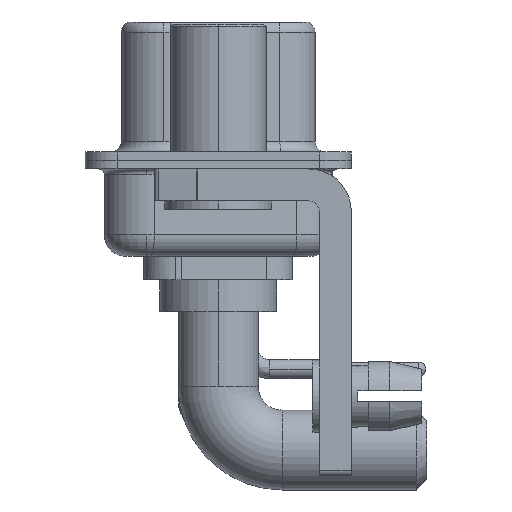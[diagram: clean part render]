
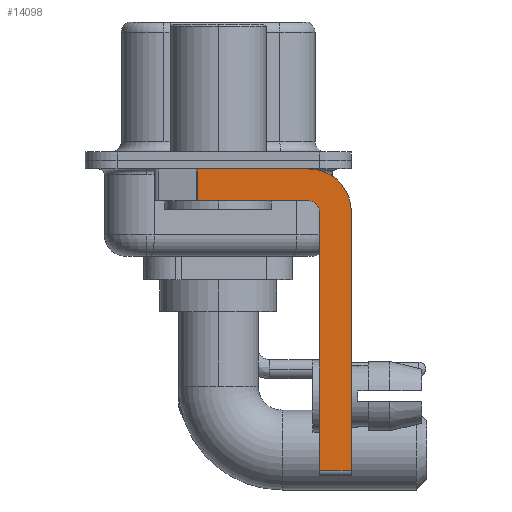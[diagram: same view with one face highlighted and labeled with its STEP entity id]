
A CAD part, left-side view. The second image highlights one B-rep face of the part: STEP entity #14098.
In plain terms, the highlighted planar face has unit normal (-1, 0, 0).
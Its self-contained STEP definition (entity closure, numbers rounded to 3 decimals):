
#633 = VERTEX_POINT ( 'NONE', #11677 ) ;
#775 = EDGE_CURVE ( 'NONE', #2592, #633, #16320, .T. ) ;
#2592 = VERTEX_POINT ( 'NONE', #19763 ) ;
#3270 = CARTESIAN_POINT ( 'NONE',  ( -2.9, -4.75, -2.4 ) ) ;
#3428 = VERTEX_POINT ( 'NONE', #3270 ) ;
#3768 = CARTESIAN_POINT ( 'NONE',  ( -2.9, -4.25, -2.4 ) ) ;
#4276 = EDGE_LOOP ( 'NONE', ( #9326, #21730, #4498, #8214, #5578, #11010, #11119, #6740 ) ) ;
#4498 = ORIENTED_EDGE ( 'NONE', *, *, #6922, .F. ) ;
#4582 = CARTESIAN_POINT ( 'NONE',  ( -2.9, -4.25, -0.4 ) ) ;
#4956 = AXIS2_PLACEMENT_3D ( 'NONE', #20406, #5187, #14983 ) ;
#5001 = CARTESIAN_POINT ( 'NONE',  ( -2.9, 0.978, -1.9 ) ) ;
#5187 = DIRECTION ( 'NONE',  ( -1., 0., 0. ) ) ;
#5353 = LINE ( 'NONE', #20832, #12167 ) ;
#5423 = CARTESIAN_POINT ( 'NONE',  ( -2.9, -4.25, -1.9 ) ) ;
#5578 = ORIENTED_EDGE ( 'NONE', *, *, #13002, .F. ) ;
#5621 = LINE ( 'NONE', #15037, #17516 ) ;
#5906 = PLANE ( 'NONE',  #6589 ) ;
#6129 = CARTESIAN_POINT ( 'NONE',  ( -2.9, -4.25, -2.4 ) ) ;
#6556 = VECTOR ( 'NONE', #11486, 1000. ) ;
#6589 = AXIS2_PLACEMENT_3D ( 'NONE', #3768, #19497, #24944 ) ;
#6740 = ORIENTED_EDGE ( 'NONE', *, *, #20470, .F. ) ;
#6922 = EDGE_CURVE ( 'NONE', #8669, #633, #5353, .T. ) ;
#7540 = LINE ( 'NONE', #13399, #6556 ) ;
#7844 = VECTOR ( 'NONE', #14550, 1000. ) ;
#8214 = ORIENTED_EDGE ( 'NONE', *, *, #13519, .F. ) ;
#8218 = EDGE_CURVE ( 'NONE', #18085, #17598, #7540, .T. ) ;
#8669 = VERTEX_POINT ( 'NONE', #5423 ) ;
#9326 = ORIENTED_EDGE ( 'NONE', *, *, #13284, .F. ) ;
#9470 = FACE_OUTER_BOUND ( 'NONE', #4276, .T. ) ;
#10222 = LINE ( 'NONE', #21998, #17088 ) ;
#10556 = VERTEX_POINT ( 'NONE', #4582 ) ;
#11010 = ORIENTED_EDGE ( 'NONE', *, *, #8218, .T. ) ;
#11119 = ORIENTED_EDGE ( 'NONE', *, *, #16963, .F. ) ;
#11486 = DIRECTION ( 'NONE',  ( 0., -1., 0. ) ) ;
#11677 = CARTESIAN_POINT ( 'NONE',  ( -2.9, 0.978, -1.9 ) ) ;
#12007 = CIRCLE ( 'NONE', #22108, 2. ) ;
#12167 = VECTOR ( 'NONE', #18302, 1000. ) ;
#13002 = EDGE_CURVE ( 'NONE', #18085, #3428, #10222, .T. ) ;
#13284 = EDGE_CURVE ( 'NONE', #2592, #10556, #5621, .T. ) ;
#13399 = CARTESIAN_POINT ( 'NONE',  ( -2.9, -4.25, -14.55 ) ) ;
#13519 = EDGE_CURVE ( 'NONE', #3428, #8669, #15122, .T. ) ;
#13647 = DIRECTION ( 'NONE',  ( 0., 0., -1. ) ) ;
#13901 = DIRECTION ( 'NONE',  ( 1., 0., 0. ) ) ;
#14098 = ADVANCED_FACE ( 'NONE', ( #9470 ), #5906, .F. ) ;
#14173 = DIRECTION ( 'NONE',  ( 0., 0., 1. ) ) ;
#14500 = LINE ( 'NONE', #22211, #17195 ) ;
#14550 = DIRECTION ( 'NONE',  ( 0., 0., -1. ) ) ;
#14983 = DIRECTION ( 'NONE',  ( 0., 0., 1. ) ) ;
#15037 = CARTESIAN_POINT ( 'NONE',  ( -2.9, 3., -0.4 ) ) ;
#15122 = CIRCLE ( 'NONE', #4956, 0.5 ) ;
#16320 = LINE ( 'NONE', #5001, #7844 ) ;
#16439 = VERTEX_POINT ( 'NONE', #16442 ) ;
#16442 = CARTESIAN_POINT ( 'NONE',  ( -2.9, -6.25, -2.4 ) ) ;
#16963 = EDGE_CURVE ( 'NONE', #16439, #17598, #14500, .T. ) ;
#17088 = VECTOR ( 'NONE', #14173, 1000. ) ;
#17135 = DIRECTION ( 'NONE',  ( 0., 0., -1. ) ) ;
#17195 = VECTOR ( 'NONE', #17135, 1000. ) ;
#17516 = VECTOR ( 'NONE', #23265, 1000. ) ;
#17598 = VERTEX_POINT ( 'NONE', #23324 ) ;
#18085 = VERTEX_POINT ( 'NONE', #23426 ) ;
#18302 = DIRECTION ( 'NONE',  ( 0., 1., 0. ) ) ;
#19497 = DIRECTION ( 'NONE',  ( 1., 0., 0. ) ) ;
#19763 = CARTESIAN_POINT ( 'NONE',  ( -2.9, 0.978, -0.4 ) ) ;
#20406 = CARTESIAN_POINT ( 'NONE',  ( -2.9, -4.25, -2.4 ) ) ;
#20470 = EDGE_CURVE ( 'NONE', #10556, #16439, #12007, .T. ) ;
#20832 = CARTESIAN_POINT ( 'NONE',  ( -2.9, -4.25, -1.9 ) ) ;
#21730 = ORIENTED_EDGE ( 'NONE', *, *, #775, .T. ) ;
#21998 = CARTESIAN_POINT ( 'NONE',  ( -2.9, -4.75, -14.8 ) ) ;
#22108 = AXIS2_PLACEMENT_3D ( 'NONE', #6129, #13901, #13647 ) ;
#22211 = CARTESIAN_POINT ( 'NONE',  ( -2.9, -6.25, -2.4 ) ) ;
#23265 = DIRECTION ( 'NONE',  ( 0., -1., 0. ) ) ;
#23324 = CARTESIAN_POINT ( 'NONE',  ( -2.9, -6.25, -14.55 ) ) ;
#23426 = CARTESIAN_POINT ( 'NONE',  ( -2.9, -4.75, -14.55 ) ) ;
#24944 = DIRECTION ( 'NONE',  ( 0., 0., -1. ) ) ;
